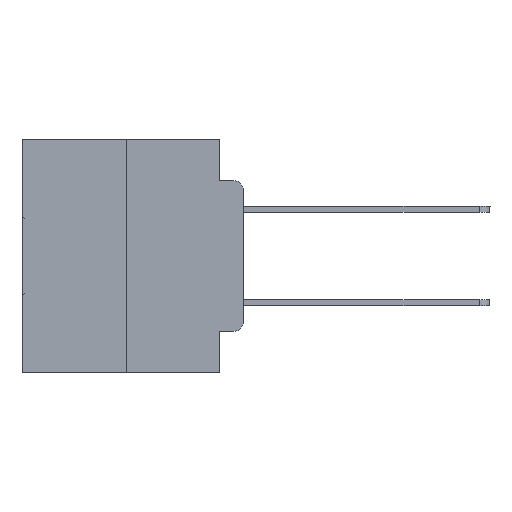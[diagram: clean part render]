
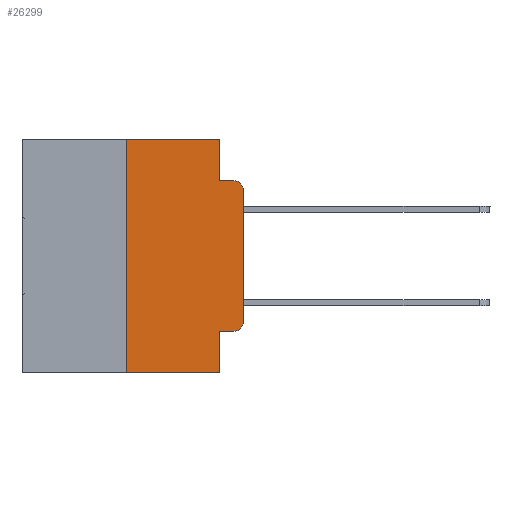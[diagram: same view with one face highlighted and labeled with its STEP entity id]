
A CAD part, left-side view. The second image highlights one B-rep face of the part: STEP entity #26299.
In plain terms, the highlighted planar face has unit normal (-1, 0, 0).
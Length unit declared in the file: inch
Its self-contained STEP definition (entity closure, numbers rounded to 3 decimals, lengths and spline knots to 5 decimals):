
#14 = DIRECTION ( 'NONE',  ( 0., 0., 1. ) ) ;
#614 = ORIENTED_EDGE ( 'NONE', *, *, #30872, .F. ) ;
#1224 = CARTESIAN_POINT ( 'NONE',  ( 0., 0.051, -0.5 ) ) ;
#1618 = VERTEX_POINT ( 'NONE', #1224 ) ;
#1874 = EDGE_CURVE ( 'NONE', #18339, #1618, #18195, .T. ) ;
#2549 = CARTESIAN_POINT ( 'NONE',  ( 0., 0.25, 0. ) ) ;
#3067 = ORIENTED_EDGE ( 'NONE', *, *, #25526, .F. ) ;
#3779 = CARTESIAN_POINT ( 'NONE',  ( 0., 0.02, -0.3915 ) ) ;
#3908 = ORIENTED_EDGE ( 'NONE', *, *, #29408, .T. ) ;
#3945 = VECTOR ( 'NONE', #14, 39.37008 ) ;
#3998 = VECTOR ( 'NONE', #5624, 39.37008 ) ;
#4785 = LINE ( 'NONE', #10489, #3998 ) ;
#4788 = LINE ( 'NONE', #20263, #22368 ) ;
#5624 = DIRECTION ( 'NONE',  ( 0., -1., 0. ) ) ;
#5932 = VERTEX_POINT ( 'NONE', #11709 ) ;
#6009 = ORIENTED_EDGE ( 'NONE', *, *, #26189, .T. ) ;
#6123 = ORIENTED_EDGE ( 'NONE', *, *, #30287, .F. ) ;
#6288 = FACE_OUTER_BOUND ( 'NONE', #29343, .T. ) ;
#6297 = DIRECTION ( 'NONE',  ( 0., 0., -1. ) ) ;
#6345 = PLANE ( 'NONE',  #20352 ) ;
#8169 = ORIENTED_EDGE ( 'NONE', *, *, #18355, .F. ) ;
#8817 = DIRECTION ( 'NONE',  ( 1., 0., 0. ) ) ;
#10489 = CARTESIAN_POINT ( 'NONE',  ( 0., 0.051, -0.0885 ) ) ;
#10902 = DIRECTION ( 'NONE',  ( 0., -1., 0. ) ) ;
#10956 = DIRECTION ( 'NONE',  ( 0., 0., -1. ) ) ;
#11347 = ORIENTED_EDGE ( 'NONE', *, *, #1874, .T. ) ;
#11709 = CARTESIAN_POINT ( 'NONE',  ( 0., 0.051, -0.0885 ) ) ;
#12002 = LINE ( 'NONE', #2549, #3945 ) ;
#12178 = DIRECTION ( 'NONE',  ( -1., 0., 0. ) ) ;
#12374 = VECTOR ( 'NONE', #13002, 39.37008 ) ;
#12601 = VECTOR ( 'NONE', #10902, 39.37008 ) ;
#13002 = DIRECTION ( 'NONE',  ( 0., -1., 0. ) ) ;
#13196 = CIRCLE ( 'NONE', #21127, 0.02 ) ;
#13229 = ORIENTED_EDGE ( 'NONE', *, *, #14482, .T. ) ;
#13795 = VECTOR ( 'NONE', #24927, 39.37008 ) ;
#14006 = LINE ( 'NONE', #27442, #31207 ) ;
#14482 = EDGE_CURVE ( 'NONE', #27982, #17178, #13196, .T. ) ;
#15188 = ORIENTED_EDGE ( 'NONE', *, *, #21354, .T. ) ;
#15318 = CARTESIAN_POINT ( 'NONE',  ( 0., 0.473, 0. ) ) ;
#15646 = DIRECTION ( 'NONE',  ( 0., 0., -1. ) ) ;
#15699 = VERTEX_POINT ( 'NONE', #23548 ) ;
#15729 = VECTOR ( 'NONE', #20251, 39.37008 ) ;
#16799 = ORIENTED_EDGE ( 'NONE', *, *, #19916, .F. ) ;
#17178 = VERTEX_POINT ( 'NONE', #27716 ) ;
#17503 = AXIS2_PLACEMENT_3D ( 'NONE', #3779, #20597, #6297 ) ;
#17974 = VERTEX_POINT ( 'NONE', #19063 ) ;
#18195 = LINE ( 'NONE', #29075, #12601 ) ;
#18339 = VERTEX_POINT ( 'NONE', #27328 ) ;
#18355 = EDGE_CURVE ( 'NONE', #15699, #1618, #14006, .T. ) ;
#18678 = LINE ( 'NONE', #24865, #15729 ) ;
#19056 = VERTEX_POINT ( 'NONE', #27619 ) ;
#19063 = CARTESIAN_POINT ( 'NONE',  ( 0., 0.02, -0.4115 ) ) ;
#19916 = EDGE_CURVE ( 'NONE', #18339, #20709, #12002, .T. ) ;
#20251 = DIRECTION ( 'NONE',  ( 0., -1., 0. ) ) ;
#20263 = CARTESIAN_POINT ( 'NONE',  ( 0., 0.051, 0. ) ) ;
#20352 = AXIS2_PLACEMENT_3D ( 'NONE', #30024, #8817, #25370 ) ;
#20597 = DIRECTION ( 'NONE',  ( -1., 0., 0. ) ) ;
#20709 = VERTEX_POINT ( 'NONE', #29519 ) ;
#20731 = CARTESIAN_POINT ( 'NONE',  ( 0., 0., -0.3915 ) ) ;
#20903 = VERTEX_POINT ( 'NONE', #20731 ) ;
#21127 = AXIS2_PLACEMENT_3D ( 'NONE', #26279, #12178, #28680 ) ;
#21354 = EDGE_CURVE ( 'NONE', #20903, #27982, #26262, .T. ) ;
#22368 = VECTOR ( 'NONE', #15646, 39.37008 ) ;
#23548 = CARTESIAN_POINT ( 'NONE',  ( 0., 0.051, -0.4115 ) ) ;
#24178 = LINE ( 'NONE', #15318, #12374 ) ;
#24865 = CARTESIAN_POINT ( 'NONE',  ( 0., 0.051, -0.4115 ) ) ;
#24927 = DIRECTION ( 'NONE',  ( 0., 0., 1. ) ) ;
#25370 = DIRECTION ( 'NONE',  ( 0., 0., -1. ) ) ;
#25526 = EDGE_CURVE ( 'NONE', #5932, #17178, #4785, .T. ) ;
#26189 = EDGE_CURVE ( 'NONE', #15699, #17974, #18678, .T. ) ;
#26199 = CIRCLE ( 'NONE', #17503, 0.02 ) ;
#26262 = LINE ( 'NONE', #29596, #13795 ) ;
#26279 = CARTESIAN_POINT ( 'NONE',  ( 0., 0.02, -0.1085 ) ) ;
#26299 = ADVANCED_FACE ( 'NONE', ( #6288 ), #6345, .F. ) ;
#27328 = CARTESIAN_POINT ( 'NONE',  ( 0., 0.25, -0.5 ) ) ;
#27442 = CARTESIAN_POINT ( 'NONE',  ( 0., 0.051, 0. ) ) ;
#27619 = CARTESIAN_POINT ( 'NONE',  ( 0., 0.051, 0. ) ) ;
#27716 = CARTESIAN_POINT ( 'NONE',  ( 0., 0.02, -0.0885 ) ) ;
#27982 = VERTEX_POINT ( 'NONE', #31068 ) ;
#28680 = DIRECTION ( 'NONE',  ( 0., 0., -1. ) ) ;
#29075 = CARTESIAN_POINT ( 'NONE',  ( 0., 0.473, -0.5 ) ) ;
#29343 = EDGE_LOOP ( 'NONE', ( #15188, #13229, #3067, #6123, #614, #16799, #11347, #8169, #6009, #3908 ) ) ;
#29408 = EDGE_CURVE ( 'NONE', #17974, #20903, #26199, .T. ) ;
#29519 = CARTESIAN_POINT ( 'NONE',  ( 0., 0.25, 0. ) ) ;
#29596 = CARTESIAN_POINT ( 'NONE',  ( 0., 0., 0. ) ) ;
#30024 = CARTESIAN_POINT ( 'NONE',  ( 0., 0.473, 0. ) ) ;
#30287 = EDGE_CURVE ( 'NONE', #19056, #5932, #4788, .T. ) ;
#30872 = EDGE_CURVE ( 'NONE', #20709, #19056, #24178, .T. ) ;
#31068 = CARTESIAN_POINT ( 'NONE',  ( 0., 0., -0.1085 ) ) ;
#31207 = VECTOR ( 'NONE', #10956, 39.37008 ) ;
